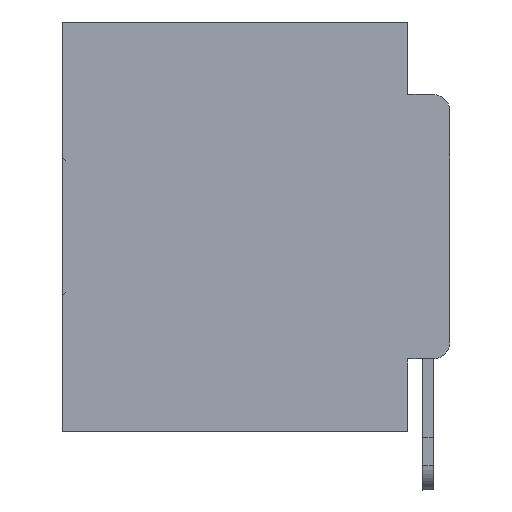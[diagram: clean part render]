
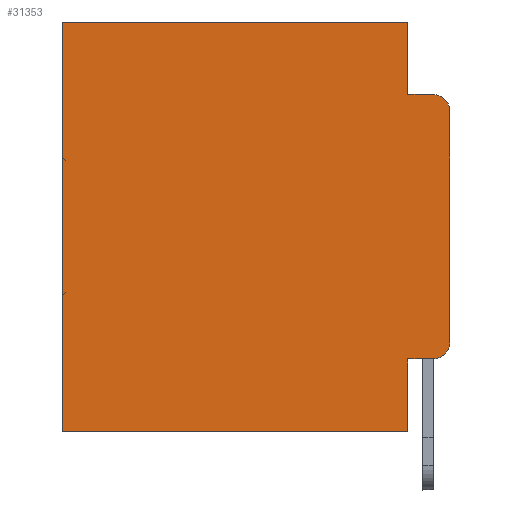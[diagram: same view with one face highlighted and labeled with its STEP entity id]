
A CAD part, left-side view. The second image highlights one B-rep face of the part: STEP entity #31353.
In plain terms, the highlighted planar face has unit normal (-1, 0, 0).
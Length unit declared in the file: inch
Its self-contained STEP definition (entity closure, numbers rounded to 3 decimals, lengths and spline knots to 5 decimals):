
#592 = LINE ( 'NONE', #18616, #29292 ) ;
#711 = CARTESIAN_POINT ( 'NONE',  ( 0.298, 0.051, 0. ) ) ;
#866 = CARTESIAN_POINT ( 'NONE',  ( 0.298, 0., 0. ) ) ;
#1869 = ORIENTED_EDGE ( 'NONE', *, *, #3690, .T. ) ;
#2606 = DIRECTION ( 'NONE',  ( 0., 1., 0. ) ) ;
#2867 = CARTESIAN_POINT ( 'NONE',  ( 0.298, 0.051, -0.5 ) ) ;
#3255 = DIRECTION ( 'NONE',  ( 0., 0., -1. ) ) ;
#3681 = ORIENTED_EDGE ( 'NONE', *, *, #14262, .T. ) ;
#3690 = EDGE_CURVE ( 'NONE', #25483, #4304, #13802, .T. ) ;
#3722 = CARTESIAN_POINT ( 'NONE',  ( 0.298, 0.051, 0. ) ) ;
#4304 = VERTEX_POINT ( 'NONE', #31246 ) ;
#4377 = VECTOR ( 'NONE', #27177, 39.37008 ) ;
#4461 = ORIENTED_EDGE ( 'NONE', *, *, #28719, .F. ) ;
#5223 = DIRECTION ( 'NONE',  ( 0., 0., -1. ) ) ;
#5614 = ORIENTED_EDGE ( 'NONE', *, *, #28919, .F. ) ;
#6060 = VECTOR ( 'NONE', #22639, 39.37008 ) ;
#6410 = LINE ( 'NONE', #3722, #17549 ) ;
#6547 = VERTEX_POINT ( 'NONE', #12839 ) ;
#6680 = VERTEX_POINT ( 'NONE', #13485 ) ;
#6926 = CARTESIAN_POINT ( 'NONE',  ( 0.298, 0.473, -0.5 ) ) ;
#7898 = DIRECTION ( 'NONE',  ( 0., 0., -1. ) ) ;
#7926 = ORIENTED_EDGE ( 'NONE', *, *, #20110, .F. ) ;
#8932 = ORIENTED_EDGE ( 'NONE', *, *, #16569, .F. ) ;
#8939 = DIRECTION ( 'NONE',  ( 0., -1., 0. ) ) ;
#9606 = EDGE_CURVE ( 'NONE', #25483, #6547, #15232, .T. ) ;
#9639 = AXIS2_PLACEMENT_3D ( 'NONE', #10809, #15397, #7898 ) ;
#9924 = VECTOR ( 'NONE', #17247, 39.37008 ) ;
#10564 = DIRECTION ( 'NONE',  ( 1., 0., 0. ) ) ;
#10687 = LINE ( 'NONE', #22922, #14240 ) ;
#10809 = CARTESIAN_POINT ( 'NONE',  ( 0.298, 0.02, -0.1085 ) ) ;
#10981 = DIRECTION ( 'NONE',  ( 0., 0., -1. ) ) ;
#12311 = LINE ( 'NONE', #22370, #9924 ) ;
#12335 = LINE ( 'NONE', #22042, #4377 ) ;
#12839 = CARTESIAN_POINT ( 'NONE',  ( 0.298, 0., -0.3915 ) ) ;
#12967 = LINE ( 'NONE', #24284, #19702 ) ;
#13448 = DIRECTION ( 'NONE',  ( -1., 0., 0. ) ) ;
#13485 = CARTESIAN_POINT ( 'NONE',  ( 0.298, 0.051, -0.0885 ) ) ;
#13802 = CIRCLE ( 'NONE', #9639, 0.02 ) ;
#13882 = EDGE_CURVE ( 'NONE', #27326, #27935, #12335, .T. ) ;
#14240 = VECTOR ( 'NONE', #5223, 39.37008 ) ;
#14262 = EDGE_CURVE ( 'NONE', #27935, #6547, #29448, .T. ) ;
#14550 = VECTOR ( 'NONE', #2606, 39.37008 ) ;
#14814 = ORIENTED_EDGE ( 'NONE', *, *, #13882, .T. ) ;
#14950 = LINE ( 'NONE', #25669, #14550 ) ;
#15232 = LINE ( 'NONE', #17528, #6060 ) ;
#15397 = DIRECTION ( 'NONE',  ( -1., 0., 0. ) ) ;
#16569 = EDGE_CURVE ( 'NONE', #27326, #29529, #592, .T. ) ;
#17176 = FACE_OUTER_BOUND ( 'NONE', #24403, .T. ) ;
#17223 = CARTESIAN_POINT ( 'NONE',  ( 0.298, 0., -0.1085 ) ) ;
#17247 = DIRECTION ( 'NONE',  ( 0., 1., 0. ) ) ;
#17528 = CARTESIAN_POINT ( 'NONE',  ( 0.298, 0., 0. ) ) ;
#17549 = VECTOR ( 'NONE', #10981, 39.37008 ) ;
#18151 = CARTESIAN_POINT ( 'NONE',  ( 0.298, 0.473, 0. ) ) ;
#18463 = VERTEX_POINT ( 'NONE', #18151 ) ;
#18554 = DIRECTION ( 'NONE',  ( 0., 0., -1. ) ) ;
#18616 = CARTESIAN_POINT ( 'NONE',  ( 0.298, 0.051, 0. ) ) ;
#18617 = ORIENTED_EDGE ( 'NONE', *, *, #9606, .F. ) ;
#19702 = VECTOR ( 'NONE', #8939, 39.37008 ) ;
#20110 = EDGE_CURVE ( 'NONE', #23194, #6680, #6410, .T. ) ;
#20289 = AXIS2_PLACEMENT_3D ( 'NONE', #866, #10564, #28397 ) ;
#20398 = EDGE_CURVE ( 'NONE', #23194, #18463, #12311, .T. ) ;
#20647 = EDGE_CURVE ( 'NONE', #18463, #30930, #10687, .T. ) ;
#20900 = PLANE ( 'NONE',  #20289 ) ;
#22042 = CARTESIAN_POINT ( 'NONE',  ( 0.298, 0.051, -0.4115 ) ) ;
#22367 = ORIENTED_EDGE ( 'NONE', *, *, #20398, .T. ) ;
#22370 = CARTESIAN_POINT ( 'NONE',  ( 0.298, 0., 0. ) ) ;
#22639 = DIRECTION ( 'NONE',  ( 0., 0., -1. ) ) ;
#22922 = CARTESIAN_POINT ( 'NONE',  ( 0.298, 0.473, 0. ) ) ;
#23194 = VERTEX_POINT ( 'NONE', #711 ) ;
#24284 = CARTESIAN_POINT ( 'NONE',  ( 0.298, 0.051, -0.0885 ) ) ;
#24403 = EDGE_LOOP ( 'NONE', ( #18617, #1869, #5614, #7926, #22367, #24915, #4461, #8932, #14814, #3681 ) ) ;
#24915 = ORIENTED_EDGE ( 'NONE', *, *, #20647, .T. ) ;
#25137 = CARTESIAN_POINT ( 'NONE',  ( 0.298, 0.02, -0.4115 ) ) ;
#25163 = CARTESIAN_POINT ( 'NONE',  ( 0.298, 0.051, -0.4115 ) ) ;
#25483 = VERTEX_POINT ( 'NONE', #17223 ) ;
#25669 = CARTESIAN_POINT ( 'NONE',  ( 0.298, 0., -0.5 ) ) ;
#27177 = DIRECTION ( 'NONE',  ( 0., -1., 0. ) ) ;
#27326 = VERTEX_POINT ( 'NONE', #25163 ) ;
#27935 = VERTEX_POINT ( 'NONE', #25137 ) ;
#28397 = DIRECTION ( 'NONE',  ( 0., 0., -1. ) ) ;
#28708 = CARTESIAN_POINT ( 'NONE',  ( 0.298, 0.02, -0.3915 ) ) ;
#28719 = EDGE_CURVE ( 'NONE', #29529, #30930, #14950, .T. ) ;
#28919 = EDGE_CURVE ( 'NONE', #6680, #4304, #12967, .T. ) ;
#29292 = VECTOR ( 'NONE', #3255, 39.37008 ) ;
#29448 = CIRCLE ( 'NONE', #31619, 0.02 ) ;
#29529 = VERTEX_POINT ( 'NONE', #2867 ) ;
#30930 = VERTEX_POINT ( 'NONE', #6926 ) ;
#31246 = CARTESIAN_POINT ( 'NONE',  ( 0.298, 0.02, -0.0885 ) ) ;
#31353 = ADVANCED_FACE ( 'NONE', ( #17176 ), #20900, .F. ) ;
#31619 = AXIS2_PLACEMENT_3D ( 'NONE', #28708, #13448, #18554 ) ;
